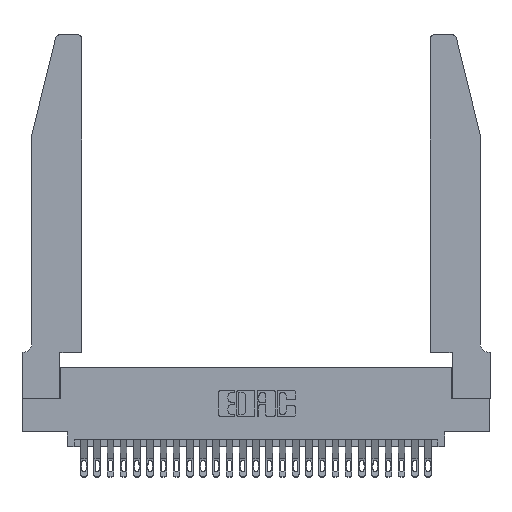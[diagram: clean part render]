
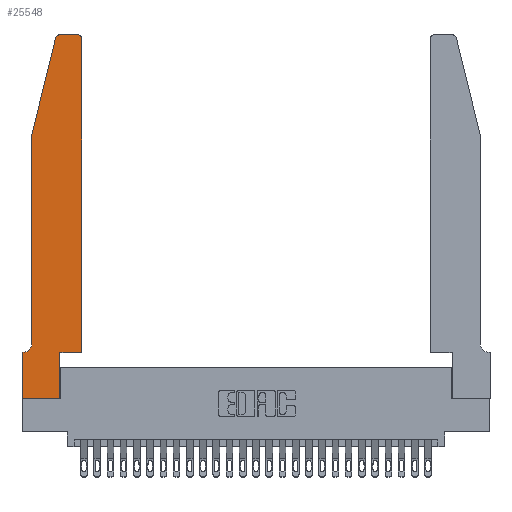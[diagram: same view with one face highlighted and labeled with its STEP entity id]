
A CAD part, top view. The second image highlights one B-rep face of the part: STEP entity #25548.
In plain terms, the highlighted planar face has unit normal (0, 0, 1).
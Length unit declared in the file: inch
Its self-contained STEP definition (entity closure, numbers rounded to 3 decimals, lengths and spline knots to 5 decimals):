
#729 = VERTEX_POINT ( 'NONE', #16008 ) ;
#886 = DIRECTION ( 'NONE',  ( 0., -1., 0. ) ) ;
#1403 = DIRECTION ( 'NONE',  ( 1., 0., 0. ) ) ;
#2504 = VECTOR ( 'NONE', #24868, 39.37008 ) ;
#2563 = DIRECTION ( 'NONE',  ( 1., 0., 0. ) ) ;
#3164 = ORIENTED_EDGE ( 'NONE', *, *, #4942, .T. ) ;
#3245 = ORIENTED_EDGE ( 'NONE', *, *, #22398, .T. ) ;
#3846 = ORIENTED_EDGE ( 'NONE', *, *, #10419, .T. ) ;
#3960 = LINE ( 'NONE', #13907, #26603 ) ;
#4149 = CARTESIAN_POINT ( 'NONE',  ( 0.4505, 2.72, 0.37 ) ) ;
#4376 = EDGE_CURVE ( 'NONE', #6568, #729, #7681, .T. ) ;
#4569 = CARTESIAN_POINT ( 'NONE',  ( 0.0055, 0.35, 0.37 ) ) ;
#4942 = EDGE_CURVE ( 'NONE', #18622, #17835, #14188, .T. ) ;
#5186 = CIRCLE ( 'NONE', #15766, 0.03 ) ;
#5454 = ORIENTED_EDGE ( 'NONE', *, *, #13326, .T. ) ;
#5649 = AXIS2_PLACEMENT_3D ( 'NONE', #15996, #24624, #15892 ) ;
#5910 = CIRCLE ( 'NONE', #8808, 0.03 ) ;
#6206 = ORIENTED_EDGE ( 'NONE', *, *, #4376, .T. ) ;
#6520 = CARTESIAN_POINT ( 'NONE',  ( 0.0755, 0.42, 0.37 ) ) ;
#6568 = VERTEX_POINT ( 'NONE', #7951 ) ;
#6817 = CARTESIAN_POINT ( 'NONE',  ( 0.0755, 2., 0.37 ) ) ;
#7115 = DIRECTION ( 'NONE',  ( 0., 0., -1. ) ) ;
#7308 = CARTESIAN_POINT ( 'NONE',  ( 0.0755, 0.35, 0.37 ) ) ;
#7681 = LINE ( 'NONE', #13317, #7719 ) ;
#7719 = VECTOR ( 'NONE', #2563, 39.37008 ) ;
#7951 = CARTESIAN_POINT ( 'NONE',  ( 0., 0., 0.37 ) ) ;
#8268 = LINE ( 'NONE', #18003, #19251 ) ;
#8566 = VERTEX_POINT ( 'NONE', #12600 ) ;
#8808 = AXIS2_PLACEMENT_3D ( 'NONE', #14254, #16773, #25574 ) ;
#9435 = CARTESIAN_POINT ( 'NONE',  ( 0., 0., 0.37 ) ) ;
#9453 = FACE_OUTER_BOUND ( 'NONE', #28220, .T. ) ;
#10100 = LINE ( 'NONE', #9435, #10759 ) ;
#10226 = DIRECTION ( 'NONE',  ( -0.239, -0.971, 0. ) ) ;
#10312 = CARTESIAN_POINT ( 'NONE',  ( 0.4205, 2.75, 0.37 ) ) ;
#10419 = EDGE_CURVE ( 'NONE', #22933, #25830, #3960, .T. ) ;
#10596 = ORIENTED_EDGE ( 'NONE', *, *, #13080, .T. ) ;
#10649 = VERTEX_POINT ( 'NONE', #10312 ) ;
#10759 = VECTOR ( 'NONE', #886, 39.37008 ) ;
#10813 = DIRECTION ( 'NONE',  ( -1., 0., 0. ) ) ;
#11215 = EDGE_CURVE ( 'NONE', #8566, #6568, #10100, .T. ) ;
#11467 = PLANE ( 'NONE',  #5649 ) ;
#11662 = CARTESIAN_POINT ( 'NONE',  ( 0.4505, 0.35, 0.37 ) ) ;
#12101 = EDGE_CURVE ( 'NONE', #16961, #8566, #20754, .T. ) ;
#12527 = DIRECTION ( 'NONE',  ( 1., 0., 0. ) ) ;
#12600 = CARTESIAN_POINT ( 'NONE',  ( 0., 0.35, 0.37 ) ) ;
#13080 = EDGE_CURVE ( 'NONE', #17835, #10649, #5910, .T. ) ;
#13317 = CARTESIAN_POINT ( 'NONE',  ( 0., 0., 0.37 ) ) ;
#13326 = EDGE_CURVE ( 'NONE', #20683, #27781, #5186, .T. ) ;
#13456 = DIRECTION ( 'NONE',  ( 0., -1., 0. ) ) ;
#13662 = LINE ( 'NONE', #19348, #16093 ) ;
#13907 = CARTESIAN_POINT ( 'NONE',  ( 0.0755, 2., 0.37 ) ) ;
#14188 = LINE ( 'NONE', #19896, #25865 ) ;
#14254 = CARTESIAN_POINT ( 'NONE',  ( 0.4205, 2.72, 0.37 ) ) ;
#14759 = CARTESIAN_POINT ( 'NONE',  ( 0.4505, 0.35, 0.37 ) ) ;
#14830 = CARTESIAN_POINT ( 'NONE',  ( 0.284, 2.72, 0.37 ) ) ;
#14847 = CARTESIAN_POINT ( 'NONE',  ( 0.2865, 0.35, 0.37 ) ) ;
#15766 = AXIS2_PLACEMENT_3D ( 'NONE', #14830, #27768, #12527 ) ;
#15892 = DIRECTION ( 'NONE',  ( 1., 0., 0. ) ) ;
#15996 = CARTESIAN_POINT ( 'NONE',  ( 0., 0.35, 0.37 ) ) ;
#16008 = CARTESIAN_POINT ( 'NONE',  ( 0.2865, 0., 0.37 ) ) ;
#16093 = VECTOR ( 'NONE', #10226, 39.37008 ) ;
#16773 = DIRECTION ( 'NONE',  ( 0., 0., 1. ) ) ;
#16961 = VERTEX_POINT ( 'NONE', #4569 ) ;
#17136 = ORIENTED_EDGE ( 'NONE', *, *, #18789, .T. ) ;
#17333 = ORIENTED_EDGE ( 'NONE', *, *, #11215, .T. ) ;
#17423 = ORIENTED_EDGE ( 'NONE', *, *, #12101, .T. ) ;
#17457 = EDGE_CURVE ( 'NONE', #25830, #16961, #23010, .T. ) ;
#17835 = VERTEX_POINT ( 'NONE', #4149 ) ;
#18003 = CARTESIAN_POINT ( 'NONE',  ( 0.2865, 0.35, 0.37 ) ) ;
#18622 = VERTEX_POINT ( 'NONE', #14759 ) ;
#18740 = ORIENTED_EDGE ( 'NONE', *, *, #27911, .T. ) ;
#18789 = EDGE_CURVE ( 'NONE', #10649, #20683, #19129, .T. ) ;
#19129 = LINE ( 'NONE', #21804, #19809 ) ;
#19187 = VERTEX_POINT ( 'NONE', #14847 ) ;
#19251 = VECTOR ( 'NONE', #20781, 39.37008 ) ;
#19348 = CARTESIAN_POINT ( 'NONE',  ( 0.0755, 2., 0.37 ) ) ;
#19809 = VECTOR ( 'NONE', #10813, 39.37008 ) ;
#19896 = CARTESIAN_POINT ( 'NONE',  ( 0.4505, 0.35, 0.37 ) ) ;
#20578 = DIRECTION ( 'NONE',  ( -1., 0., 0. ) ) ;
#20683 = VERTEX_POINT ( 'NONE', #21020 ) ;
#20754 = LINE ( 'NONE', #7308, #2504 ) ;
#20781 = DIRECTION ( 'NONE',  ( 0., 1., 0. ) ) ;
#21020 = CARTESIAN_POINT ( 'NONE',  ( 0.284, 2.75, 0.37 ) ) ;
#21538 = VECTOR ( 'NONE', #1403, 39.37008 ) ;
#21803 = ORIENTED_EDGE ( 'NONE', *, *, #23918, .T. ) ;
#21804 = CARTESIAN_POINT ( 'NONE',  ( 0.2605, 2.75, 0.37 ) ) ;
#22398 = EDGE_CURVE ( 'NONE', #729, #19187, #8268, .T. ) ;
#22780 = CARTESIAN_POINT ( 'NONE',  ( 0.0055, 0.42, 0.37 ) ) ;
#22821 = CARTESIAN_POINT ( 'NONE',  ( 0.25487, 2.72718, 0.37 ) ) ;
#22933 = VERTEX_POINT ( 'NONE', #6817 ) ;
#23010 = CIRCLE ( 'NONE', #26302, 0.07 ) ;
#23918 = EDGE_CURVE ( 'NONE', #27781, #22933, #13662, .T. ) ;
#24624 = DIRECTION ( 'NONE',  ( 0., 0., 1. ) ) ;
#24868 = DIRECTION ( 'NONE',  ( -1., 0., 0. ) ) ;
#25009 = ORIENTED_EDGE ( 'NONE', *, *, #17457, .T. ) ;
#25548 = ADVANCED_FACE ( 'NONE', ( #9453 ), #11467, .T. ) ;
#25574 = DIRECTION ( 'NONE',  ( 1., 0., 0. ) ) ;
#25830 = VERTEX_POINT ( 'NONE', #6520 ) ;
#25865 = VECTOR ( 'NONE', #26674, 39.37008 ) ;
#26302 = AXIS2_PLACEMENT_3D ( 'NONE', #22780, #7115, #20578 ) ;
#26603 = VECTOR ( 'NONE', #13456, 39.37008 ) ;
#26674 = DIRECTION ( 'NONE',  ( 0., 1., 0. ) ) ;
#27768 = DIRECTION ( 'NONE',  ( 0., 0., 1. ) ) ;
#27781 = VERTEX_POINT ( 'NONE', #22821 ) ;
#27911 = EDGE_CURVE ( 'NONE', #19187, #18622, #28023, .T. ) ;
#28023 = LINE ( 'NONE', #11662, #21538 ) ;
#28220 = EDGE_LOOP ( 'NONE', ( #17136, #5454, #21803, #3846, #25009, #17423, #17333, #6206, #3245, #18740, #3164, #10596 ) ) ;
